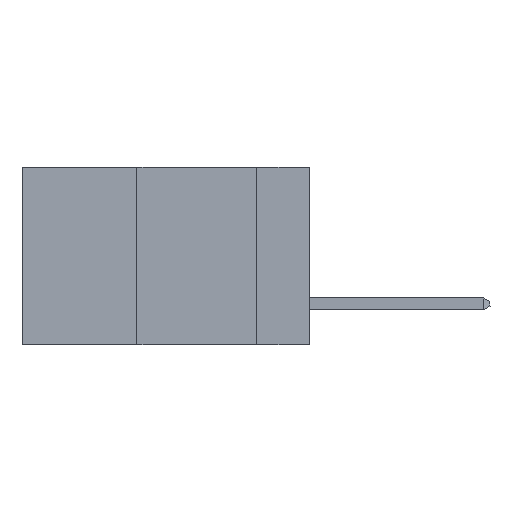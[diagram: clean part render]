
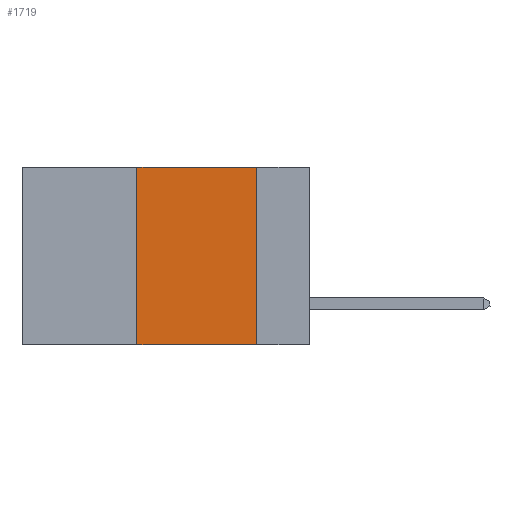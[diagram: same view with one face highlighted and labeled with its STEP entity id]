
A CAD part, left-side view. The second image highlights one B-rep face of the part: STEP entity #1719.
In plain terms, the highlighted planar face has unit normal (-1, 0, 0).
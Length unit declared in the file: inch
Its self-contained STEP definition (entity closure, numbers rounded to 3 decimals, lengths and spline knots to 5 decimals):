
#1719 = ADVANCED_FACE ( 'NONE', ( #23441 ), #7457, .F. ) ;
#1952 = VECTOR ( 'NONE', #24482, 39.37008 ) ;
#2129 = DIRECTION ( 'NONE',  ( 0., -1., 0. ) ) ;
#2514 = EDGE_CURVE ( 'NONE', #17998, #6197, #10794, .T. ) ;
#3903 = EDGE_CURVE ( 'NONE', #6197, #6769, #12243, .T. ) ;
#5431 = ORIENTED_EDGE ( 'NONE', *, *, #2514, .F. ) ;
#5519 = CARTESIAN_POINT ( 'NONE',  ( 0., 0.11, -0.37 ) ) ;
#6197 = VERTEX_POINT ( 'NONE', #22473 ) ;
#6344 = CARTESIAN_POINT ( 'NONE',  ( 0., 0.36, 0. ) ) ;
#6769 = VERTEX_POINT ( 'NONE', #5519 ) ;
#7064 = EDGE_LOOP ( 'NONE', ( #26781, #5431, #20364, #26466 ) ) ;
#7457 = PLANE ( 'NONE',  #22231 ) ;
#7926 = VECTOR ( 'NONE', #8426, 39.37008 ) ;
#8426 = DIRECTION ( 'NONE',  ( 0., 0., 1. ) ) ;
#8552 = LINE ( 'NONE', #6344, #7926 ) ;
#8586 = EDGE_CURVE ( 'NONE', #16599, #6769, #18502, .T. ) ;
#10794 = LINE ( 'NONE', #18635, #21152 ) ;
#10822 = DIRECTION ( 'NONE',  ( 0., 0., -1. ) ) ;
#11618 = CARTESIAN_POINT ( 'NONE',  ( 0., 0.6, 0. ) ) ;
#12243 = LINE ( 'NONE', #12931, #22568 ) ;
#12931 = CARTESIAN_POINT ( 'NONE',  ( 0., 0.11, 0. ) ) ;
#13739 = DIRECTION ( 'NONE',  ( 0., 0., -1. ) ) ;
#16599 = VERTEX_POINT ( 'NONE', #24274 ) ;
#17998 = VERTEX_POINT ( 'NONE', #18849 ) ;
#18315 = CARTESIAN_POINT ( 'NONE',  ( 0., 0.6, -0.37 ) ) ;
#18502 = LINE ( 'NONE', #18315, #1952 ) ;
#18635 = CARTESIAN_POINT ( 'NONE',  ( 0., 0.6, 0. ) ) ;
#18849 = CARTESIAN_POINT ( 'NONE',  ( 0., 0.36, 0. ) ) ;
#19835 = EDGE_CURVE ( 'NONE', #16599, #17998, #8552, .T. ) ;
#20364 = ORIENTED_EDGE ( 'NONE', *, *, #19835, .F. ) ;
#21152 = VECTOR ( 'NONE', #2129, 39.37008 ) ;
#22231 = AXIS2_PLACEMENT_3D ( 'NONE', #11618, #26047, #13739 ) ;
#22473 = CARTESIAN_POINT ( 'NONE',  ( 0., 0.11, 0. ) ) ;
#22568 = VECTOR ( 'NONE', #10822, 39.37008 ) ;
#23441 = FACE_OUTER_BOUND ( 'NONE', #7064, .T. ) ;
#24274 = CARTESIAN_POINT ( 'NONE',  ( 0., 0.36, -0.37 ) ) ;
#24482 = DIRECTION ( 'NONE',  ( 0., -1., 0. ) ) ;
#26047 = DIRECTION ( 'NONE',  ( 1., 0., 0. ) ) ;
#26466 = ORIENTED_EDGE ( 'NONE', *, *, #8586, .T. ) ;
#26781 = ORIENTED_EDGE ( 'NONE', *, *, #3903, .F. ) ;
